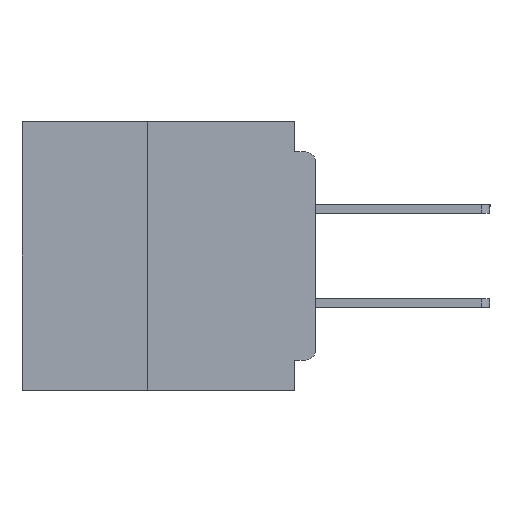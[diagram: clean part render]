
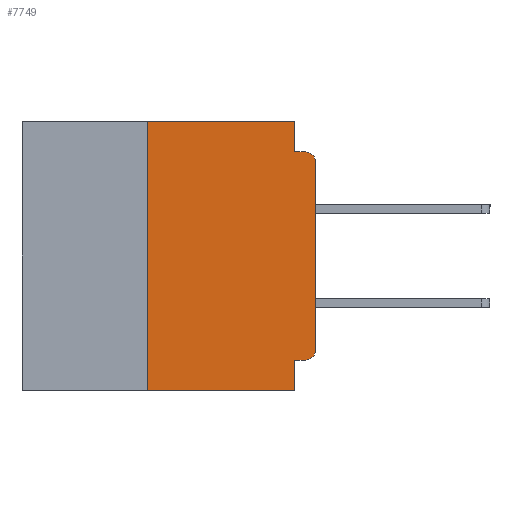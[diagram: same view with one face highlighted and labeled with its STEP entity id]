
A CAD part, left-side view. The second image highlights one B-rep face of the part: STEP entity #7749.
In plain terms, the highlighted planar face has unit normal (-1, 0, 0).
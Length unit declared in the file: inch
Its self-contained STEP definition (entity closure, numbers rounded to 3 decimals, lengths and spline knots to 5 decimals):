
#385 = CARTESIAN_POINT ( 'NONE',  ( 0., 0., -0.34 ) ) ;
#772 = CARTESIAN_POINT ( 'NONE',  ( 0., 0., 0. ) ) ;
#1104 = DIRECTION ( 'NONE',  ( 0., -1., 0. ) ) ;
#1117 = VERTEX_POINT ( 'NONE', #19385 ) ;
#2100 = CARTESIAN_POINT ( 'NONE',  ( 0., 0., -0.06 ) ) ;
#2438 = DIRECTION ( 'NONE',  ( 1., 0., 0. ) ) ;
#2520 = AXIS2_PLACEMENT_3D ( 'NONE', #30963, #4722, #35335 ) ;
#2761 = CARTESIAN_POINT ( 'NONE',  ( 0., 0., -0.355 ) ) ;
#2957 = DIRECTION ( 'NONE',  ( -1., 0., 0. ) ) ;
#4458 = CARTESIAN_POINT ( 'NONE',  ( 0., 0.437, -0.4 ) ) ;
#4722 = DIRECTION ( 'NONE',  ( -1., 0., 0. ) ) ;
#5209 = DIRECTION ( 'NONE',  ( 0., 0., 1. ) ) ;
#5787 = LINE ( 'NONE', #2761, #50952 ) ;
#6899 = EDGE_LOOP ( 'NONE', ( #12938, #15416, #50676, #39301, #22473, #14717, #25310, #38101, #10091, #47857 ) ) ;
#7561 = AXIS2_PLACEMENT_3D ( 'NONE', #50432, #2438, #33081 ) ;
#7749 = ADVANCED_FACE ( 'NONE', ( #48117 ), #28728, .F. ) ;
#8652 = VERTEX_POINT ( 'NONE', #26152 ) ;
#8819 = EDGE_CURVE ( 'NONE', #40804, #38324, #28252, .T. ) ;
#9187 = VECTOR ( 'NONE', #10527, 39.37008 ) ;
#9697 = CARTESIAN_POINT ( 'NONE',  ( 0., 0.25, 0. ) ) ;
#10091 = ORIENTED_EDGE ( 'NONE', *, *, #51387, .F. ) ;
#10527 = DIRECTION ( 'NONE',  ( 0., 0., 1. ) ) ;
#12938 = ORIENTED_EDGE ( 'NONE', *, *, #8819, .T. ) ;
#13174 = DIRECTION ( 'NONE',  ( 0., -1., 0. ) ) ;
#13581 = DIRECTION ( 'NONE',  ( 0., 0., -1. ) ) ;
#14717 = ORIENTED_EDGE ( 'NONE', *, *, #23900, .F. ) ;
#14863 = LINE ( 'NONE', #22526, #38225 ) ;
#14982 = EDGE_CURVE ( 'NONE', #27721, #8652, #45627, .T. ) ;
#15416 = ORIENTED_EDGE ( 'NONE', *, *, #51383, .T. ) ;
#15698 = CARTESIAN_POINT ( 'NONE',  ( 0., 0.031, -0.4 ) ) ;
#16494 = VECTOR ( 'NONE', #5209, 39.37008 ) ;
#16915 = VECTOR ( 'NONE', #20172, 39.37008 ) ;
#17422 = CIRCLE ( 'NONE', #34735, 0.015 ) ;
#17893 = VERTEX_POINT ( 'NONE', #50238 ) ;
#18293 = EDGE_CURVE ( 'NONE', #25821, #40804, #32351, .T. ) ;
#18803 = CARTESIAN_POINT ( 'NONE',  ( 0., 0., -0.045 ) ) ;
#19385 = CARTESIAN_POINT ( 'NONE',  ( 0., 0.25, -0.4 ) ) ;
#20172 = DIRECTION ( 'NONE',  ( 0., 0., -1. ) ) ;
#21561 = VERTEX_POINT ( 'NONE', #29795 ) ;
#21665 = VECTOR ( 'NONE', #13174, 39.37008 ) ;
#21932 = EDGE_CURVE ( 'NONE', #22052, #17893, #50412, .T. ) ;
#22052 = VERTEX_POINT ( 'NONE', #45560 ) ;
#22473 = ORIENTED_EDGE ( 'NONE', *, *, #14982, .F. ) ;
#22526 = CARTESIAN_POINT ( 'NONE',  ( 0., 0.031, 0. ) ) ;
#23900 = EDGE_CURVE ( 'NONE', #1117, #27721, #31182, .T. ) ;
#25310 = ORIENTED_EDGE ( 'NONE', *, *, #32095, .T. ) ;
#25821 = VERTEX_POINT ( 'NONE', #38176 ) ;
#26152 = CARTESIAN_POINT ( 'NONE',  ( 0., 0.031, 0. ) ) ;
#27673 = DIRECTION ( 'NONE',  ( 0., -1., 0. ) ) ;
#27721 = VERTEX_POINT ( 'NONE', #9697 ) ;
#28252 = LINE ( 'NONE', #772, #16494 ) ;
#28666 = LINE ( 'NONE', #15698, #16915 ) ;
#28728 = PLANE ( 'NONE',  #7561 ) ;
#29241 = CARTESIAN_POINT ( 'NONE',  ( 0., 0.015, -0.06 ) ) ;
#29795 = CARTESIAN_POINT ( 'NONE',  ( 0., 0.031, -0.355 ) ) ;
#30963 = CARTESIAN_POINT ( 'NONE',  ( 0., 0.015, -0.34 ) ) ;
#31182 = LINE ( 'NONE', #41217, #9187 ) ;
#32095 = EDGE_CURVE ( 'NONE', #1117, #34311, #56416, .T. ) ;
#32351 = CIRCLE ( 'NONE', #2520, 0.015 ) ;
#33081 = DIRECTION ( 'NONE',  ( 0., 0., -1. ) ) ;
#33590 = DIRECTION ( 'NONE',  ( 0., 0., -1. ) ) ;
#34029 = VECTOR ( 'NONE', #1104, 39.37008 ) ;
#34311 = VERTEX_POINT ( 'NONE', #50582 ) ;
#34735 = AXIS2_PLACEMENT_3D ( 'NONE', #29241, #2957, #33590 ) ;
#35335 = DIRECTION ( 'NONE',  ( 0., 0., -1. ) ) ;
#38005 = DIRECTION ( 'NONE',  ( 0., 1., 0. ) ) ;
#38101 = ORIENTED_EDGE ( 'NONE', *, *, #46952, .F. ) ;
#38176 = CARTESIAN_POINT ( 'NONE',  ( 0., 0.015, -0.355 ) ) ;
#38225 = VECTOR ( 'NONE', #13581, 39.37008 ) ;
#38324 = VERTEX_POINT ( 'NONE', #2100 ) ;
#39301 = ORIENTED_EDGE ( 'NONE', *, *, #46774, .F. ) ;
#40804 = VERTEX_POINT ( 'NONE', #385 ) ;
#41217 = CARTESIAN_POINT ( 'NONE',  ( 0., 0.25, -0.4 ) ) ;
#45560 = CARTESIAN_POINT ( 'NONE',  ( 0., 0.031, -0.045 ) ) ;
#45627 = LINE ( 'NONE', #53473, #34029 ) ;
#46774 = EDGE_CURVE ( 'NONE', #8652, #22052, #14863, .T. ) ;
#46952 = EDGE_CURVE ( 'NONE', #21561, #34311, #28666, .T. ) ;
#47680 = VECTOR ( 'NONE', #27673, 39.37008 ) ;
#47857 = ORIENTED_EDGE ( 'NONE', *, *, #18293, .T. ) ;
#48117 = FACE_OUTER_BOUND ( 'NONE', #6899, .T. ) ;
#50238 = CARTESIAN_POINT ( 'NONE',  ( 0., 0.015, -0.045 ) ) ;
#50412 = LINE ( 'NONE', #18803, #47680 ) ;
#50432 = CARTESIAN_POINT ( 'NONE',  ( 0., 0.437, 0. ) ) ;
#50582 = CARTESIAN_POINT ( 'NONE',  ( 0., 0.031, -0.4 ) ) ;
#50676 = ORIENTED_EDGE ( 'NONE', *, *, #21932, .F. ) ;
#50952 = VECTOR ( 'NONE', #38005, 39.37008 ) ;
#51383 = EDGE_CURVE ( 'NONE', #38324, #17893, #17422, .T. ) ;
#51387 = EDGE_CURVE ( 'NONE', #25821, #21561, #5787, .T. ) ;
#53473 = CARTESIAN_POINT ( 'NONE',  ( 0., 0.437, 0. ) ) ;
#56416 = LINE ( 'NONE', #4458, #21665 ) ;
